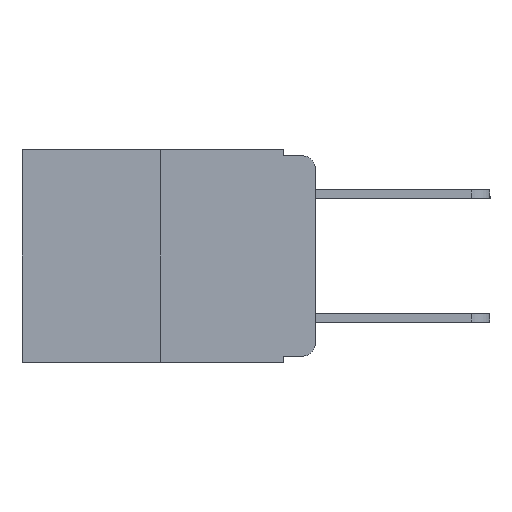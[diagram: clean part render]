
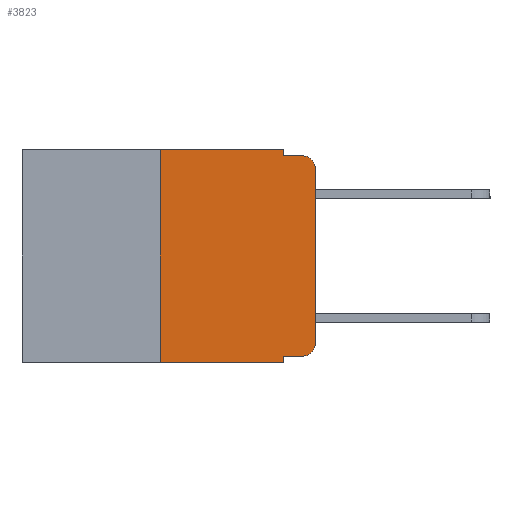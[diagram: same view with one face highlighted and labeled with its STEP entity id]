
A CAD part, left-side view. The second image highlights one B-rep face of the part: STEP entity #3823.
In plain terms, the highlighted planar face has unit normal (-1, 0, 0).
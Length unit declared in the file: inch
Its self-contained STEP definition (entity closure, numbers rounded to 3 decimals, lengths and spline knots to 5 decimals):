
#142 = DIRECTION ( 'NONE',  ( 0., -1., 0. ) ) ;
#211 = ORIENTED_EDGE ( 'NONE', *, *, #19635, .T. ) ;
#249 = EDGE_CURVE ( 'NONE', #18737, #10829, #6529, .T. ) ;
#640 = ORIENTED_EDGE ( 'NONE', *, *, #3946, .T. ) ;
#667 = ORIENTED_EDGE ( 'NONE', *, *, #3679, .F. ) ;
#897 = FACE_OUTER_BOUND ( 'NONE', #14420, .T. ) ;
#1056 = CARTESIAN_POINT ( 'NONE',  ( 0., 0.051, -0.333 ) ) ;
#1088 = VECTOR ( 'NONE', #22812, 39.37008 ) ;
#1143 = EDGE_CURVE ( 'NONE', #2893, #19373, #3677, .T. ) ;
#1338 = CIRCLE ( 'NONE', #11005, 0.02 ) ;
#1386 = DIRECTION ( 'NONE',  ( 0., 0., 1. ) ) ;
#1665 = ORIENTED_EDGE ( 'NONE', *, *, #25667, .F. ) ;
#1778 = LINE ( 'NONE', #18590, #6553 ) ;
#2160 = DIRECTION ( 'NONE',  ( 0., 0., 1. ) ) ;
#2450 = CARTESIAN_POINT ( 'NONE',  ( 0., 0., -0.03 ) ) ;
#2552 = VECTOR ( 'NONE', #2160, 39.37008 ) ;
#2805 = CARTESIAN_POINT ( 'NONE',  ( 0., 0.051, 0. ) ) ;
#2893 = VERTEX_POINT ( 'NONE', #2450 ) ;
#3369 = ORIENTED_EDGE ( 'NONE', *, *, #8456, .F. ) ;
#3677 = CIRCLE ( 'NONE', #17383, 0.02 ) ;
#3679 = EDGE_CURVE ( 'NONE', #15896, #14488, #24605, .T. ) ;
#3808 = CARTESIAN_POINT ( 'NONE',  ( 0., 0.473, 0. ) ) ;
#3823 = ADVANCED_FACE ( 'NONE', ( #897 ), #13775, .F. ) ;
#3946 = EDGE_CURVE ( 'NONE', #6315, #2893, #23707, .T. ) ;
#4940 = CARTESIAN_POINT ( 'NONE',  ( 0., 0.051, -0.333 ) ) ;
#5271 = CARTESIAN_POINT ( 'NONE',  ( 0., 0.473, 0. ) ) ;
#5398 = DIRECTION ( 'NONE',  ( 0., 0., -1. ) ) ;
#5441 = DIRECTION ( 'NONE',  ( 0., -1., 0. ) ) ;
#5556 = ORIENTED_EDGE ( 'NONE', *, *, #18467, .T. ) ;
#5704 = CARTESIAN_POINT ( 'NONE',  ( 0., 0.02, -0.03 ) ) ;
#5825 = ORIENTED_EDGE ( 'NONE', *, *, #1143, .T. ) ;
#5836 = DIRECTION ( 'NONE',  ( 0., 0., -1. ) ) ;
#6024 = DIRECTION ( 'NONE',  ( -1., 0., 0. ) ) ;
#6315 = VERTEX_POINT ( 'NONE', #12570 ) ;
#6502 = LINE ( 'NONE', #14290, #12463 ) ;
#6529 = LINE ( 'NONE', #4940, #1088 ) ;
#6553 = VECTOR ( 'NONE', #8686, 39.37008 ) ;
#6779 = ORIENTED_EDGE ( 'NONE', *, *, #12495, .F. ) ;
#7012 = CARTESIAN_POINT ( 'NONE',  ( 0., 0.051, -0.343 ) ) ;
#7720 = DIRECTION ( 'NONE',  ( 0., 0., -1. ) ) ;
#8103 = VECTOR ( 'NONE', #5441, 39.37008 ) ;
#8456 = EDGE_CURVE ( 'NONE', #18737, #12329, #12662, .T. ) ;
#8686 = DIRECTION ( 'NONE',  ( 0., 0., -1. ) ) ;
#9156 = CARTESIAN_POINT ( 'NONE',  ( 0., 0.25, 0. ) ) ;
#9595 = ORIENTED_EDGE ( 'NONE', *, *, #23050, .F. ) ;
#10829 = VERTEX_POINT ( 'NONE', #10904 ) ;
#10904 = CARTESIAN_POINT ( 'NONE',  ( 0., 0.02, -0.333 ) ) ;
#11005 = AXIS2_PLACEMENT_3D ( 'NONE', #17974, #6024, #19947 ) ;
#11301 = DIRECTION ( 'NONE',  ( 0., -1., 0. ) ) ;
#11393 = CARTESIAN_POINT ( 'NONE',  ( 0., 0.051, -0.01 ) ) ;
#12329 = VERTEX_POINT ( 'NONE', #7012 ) ;
#12463 = VECTOR ( 'NONE', #142, 39.37008 ) ;
#12495 = EDGE_CURVE ( 'NONE', #19362, #15896, #24636, .T. ) ;
#12570 = CARTESIAN_POINT ( 'NONE',  ( 0., 0., -0.313 ) ) ;
#12662 = LINE ( 'NONE', #13349, #22507 ) ;
#13349 = CARTESIAN_POINT ( 'NONE',  ( 0., 0.051, 0. ) ) ;
#13775 = PLANE ( 'NONE',  #18233 ) ;
#14167 = VECTOR ( 'NONE', #11301, 39.37008 ) ;
#14202 = CARTESIAN_POINT ( 'NONE',  ( 0., 0., 0. ) ) ;
#14290 = CARTESIAN_POINT ( 'NONE',  ( 0., 0.473, -0.343 ) ) ;
#14420 = EDGE_LOOP ( 'NONE', ( #640, #5825, #1665, #9595, #667, #6779, #5556, #3369, #25685, #211 ) ) ;
#14488 = VERTEX_POINT ( 'NONE', #2805 ) ;
#15472 = CARTESIAN_POINT ( 'NONE',  ( 0., 0.25, 0. ) ) ;
#15896 = VERTEX_POINT ( 'NONE', #9156 ) ;
#17131 = VERTEX_POINT ( 'NONE', #25838 ) ;
#17383 = AXIS2_PLACEMENT_3D ( 'NONE', #5704, #19636, #7720 ) ;
#17771 = DIRECTION ( 'NONE',  ( 1., 0., 0. ) ) ;
#17974 = CARTESIAN_POINT ( 'NONE',  ( 0., 0.02, -0.313 ) ) ;
#18233 = AXIS2_PLACEMENT_3D ( 'NONE', #3808, #17771, #5836 ) ;
#18467 = EDGE_CURVE ( 'NONE', #19362, #12329, #6502, .T. ) ;
#18590 = CARTESIAN_POINT ( 'NONE',  ( 0., 0.051, 0. ) ) ;
#18737 = VERTEX_POINT ( 'NONE', #1056 ) ;
#19302 = LINE ( 'NONE', #11393, #8103 ) ;
#19362 = VERTEX_POINT ( 'NONE', #22936 ) ;
#19373 = VERTEX_POINT ( 'NONE', #24890 ) ;
#19476 = VECTOR ( 'NONE', #1386, 39.37008 ) ;
#19635 = EDGE_CURVE ( 'NONE', #10829, #6315, #1338, .T. ) ;
#19636 = DIRECTION ( 'NONE',  ( -1., 0., 0. ) ) ;
#19947 = DIRECTION ( 'NONE',  ( 0., 0., -1. ) ) ;
#22507 = VECTOR ( 'NONE', #5398, 39.37008 ) ;
#22812 = DIRECTION ( 'NONE',  ( 0., -1., 0. ) ) ;
#22936 = CARTESIAN_POINT ( 'NONE',  ( 0., 0.25, -0.343 ) ) ;
#23050 = EDGE_CURVE ( 'NONE', #14488, #17131, #1778, .T. ) ;
#23707 = LINE ( 'NONE', #14202, #2552 ) ;
#24605 = LINE ( 'NONE', #5271, #14167 ) ;
#24636 = LINE ( 'NONE', #15472, #19476 ) ;
#24890 = CARTESIAN_POINT ( 'NONE',  ( 0., 0.02, -0.01 ) ) ;
#25667 = EDGE_CURVE ( 'NONE', #17131, #19373, #19302, .T. ) ;
#25685 = ORIENTED_EDGE ( 'NONE', *, *, #249, .T. ) ;
#25838 = CARTESIAN_POINT ( 'NONE',  ( 0., 0.051, -0.01 ) ) ;
